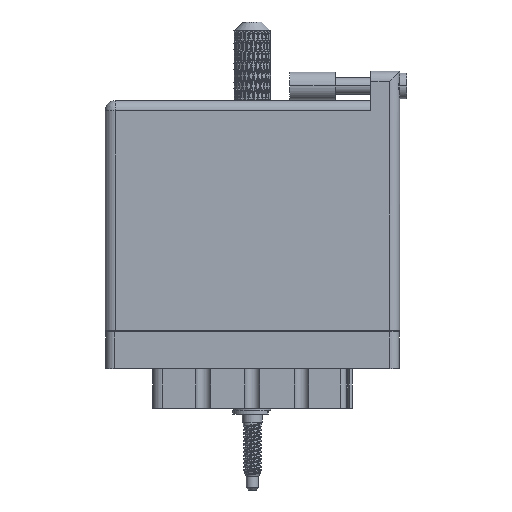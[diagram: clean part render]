
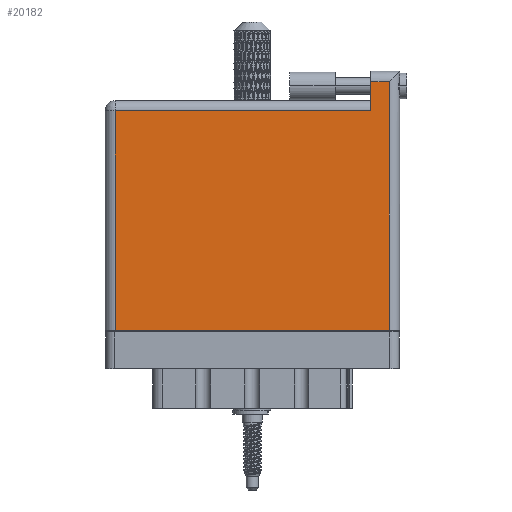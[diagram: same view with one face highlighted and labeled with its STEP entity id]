
A CAD part, front view. The second image highlights one B-rep face of the part: STEP entity #20182.
In plain terms, the highlighted face is planar.
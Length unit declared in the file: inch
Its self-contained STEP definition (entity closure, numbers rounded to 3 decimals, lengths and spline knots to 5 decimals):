
#1278 = VECTOR ( 'NONE', #25724, 39.37008 ) ;
#1497 = EDGE_CURVE ( 'NONE', #20275, #52184, #72301, .T. ) ;
#3825 = LINE ( 'NONE', #60102, #38678 ) ;
#6095 = DIRECTION ( 'NONE',  ( 0., 1., 0. ) ) ;
#7097 = LINE ( 'NONE', #106779, #92278 ) ;
#9854 = ORIENTED_EDGE ( 'NONE', *, *, #59453, .T. ) ;
#20182 = ADVANCED_FACE ( 'NONE', ( #38812 ), #42728, .F. ) ;
#20275 = VERTEX_POINT ( 'NONE', #44505 ) ;
#21572 = CARTESIAN_POINT ( 'NONE',  ( 0.07, 1.496, 0. ) ) ;
#25724 = DIRECTION ( 'NONE',  ( -1., 0., 0. ) ) ;
#35802 = VERTEX_POINT ( 'NONE', #21572 ) ;
#37406 = EDGE_LOOP ( 'NONE', ( #105704, #9854, #61619, #78210, #38801, #41204 ) ) ;
#37929 = EDGE_CURVE ( 'NONE', #42279, #100147, #76722, .T. ) ;
#38678 = VECTOR ( 'NONE', #92577, 39.37008 ) ;
#38801 = ORIENTED_EDGE ( 'NONE', *, *, #89812, .T. ) ;
#38812 = FACE_OUTER_BOUND ( 'NONE', #37406, .T. ) ;
#41204 = ORIENTED_EDGE ( 'NONE', *, *, #95743, .T. ) ;
#42261 = VECTOR ( 'NONE', #6095, 39.37008 ) ;
#42279 = VERTEX_POINT ( 'NONE', #55212 ) ;
#42728 = PLANE ( 'NONE',  #65106 ) ;
#44505 = CARTESIAN_POINT ( 'NONE',  ( 1.811, 1.696, 0. ) ) ;
#45428 = CARTESIAN_POINT ( 'NONE',  ( 1.811, 1.766, 0. ) ) ;
#51723 = DIRECTION ( 'NONE',  ( -1., 0., 0. ) ) ;
#52184 = VERTEX_POINT ( 'NONE', #92058 ) ;
#53862 = LINE ( 'NONE', #56254, #42261 ) ;
#54817 = VECTOR ( 'NONE', #60345, 39.37008 ) ;
#55212 = CARTESIAN_POINT ( 'NONE',  ( 0.07, 0., 0. ) ) ;
#56254 = CARTESIAN_POINT ( 'NONE',  ( 1.938, 1.766, 0. ) ) ;
#57408 = DIRECTION ( 'NONE',  ( 0., -1., 0. ) ) ;
#59453 = EDGE_CURVE ( 'NONE', #100147, #67659, #53862, .T. ) ;
#59639 = DIRECTION ( 'NONE',  ( 0., 0., -1. ) ) ;
#60102 = CARTESIAN_POINT ( 'NONE',  ( 0., 1.696, 0. ) ) ;
#60345 = DIRECTION ( 'NONE',  ( 1., 0., 0. ) ) ;
#61619 = ORIENTED_EDGE ( 'NONE', *, *, #105952, .T. ) ;
#62116 = CARTESIAN_POINT ( 'NONE',  ( 1.938, 1.696, 0. ) ) ;
#65106 = AXIS2_PLACEMENT_3D ( 'NONE', #68331, #59639, #51723 ) ;
#66125 = CARTESIAN_POINT ( 'NONE',  ( 0., 1.496, 0. ) ) ;
#67659 = VERTEX_POINT ( 'NONE', #62116 ) ;
#68331 = CARTESIAN_POINT ( 'NONE',  ( 0., 1.566, 0. ) ) ;
#72301 = LINE ( 'NONE', #45428, #89091 ) ;
#76710 = CARTESIAN_POINT ( 'NONE',  ( 1.938, 0., 0. ) ) ;
#76722 = LINE ( 'NONE', #92844, #54817 ) ;
#78210 = ORIENTED_EDGE ( 'NONE', *, *, #1497, .T. ) ;
#85183 = LINE ( 'NONE', #66125, #1278 ) ;
#86541 = DIRECTION ( 'NONE',  ( 0., -1., 0. ) ) ;
#89091 = VECTOR ( 'NONE', #86541, 39.37008 ) ;
#89812 = EDGE_CURVE ( 'NONE', #52184, #35802, #85183, .T. ) ;
#92058 = CARTESIAN_POINT ( 'NONE',  ( 1.811, 1.496, 0. ) ) ;
#92278 = VECTOR ( 'NONE', #57408, 39.37008 ) ;
#92577 = DIRECTION ( 'NONE',  ( -1., 0., 0. ) ) ;
#92844 = CARTESIAN_POINT ( 'NONE',  ( 0., 0., 0. ) ) ;
#95743 = EDGE_CURVE ( 'NONE', #35802, #42279, #7097, .T. ) ;
#100147 = VERTEX_POINT ( 'NONE', #76710 ) ;
#105704 = ORIENTED_EDGE ( 'NONE', *, *, #37929, .T. ) ;
#105952 = EDGE_CURVE ( 'NONE', #67659, #20275, #3825, .T. ) ;
#106779 = CARTESIAN_POINT ( 'NONE',  ( 0.07, 0., 0. ) ) ;
